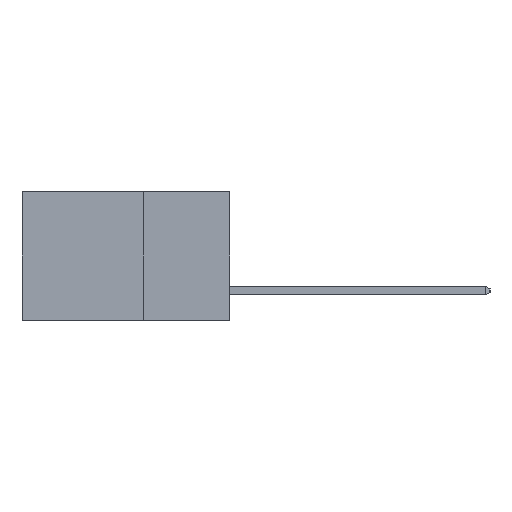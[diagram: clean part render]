
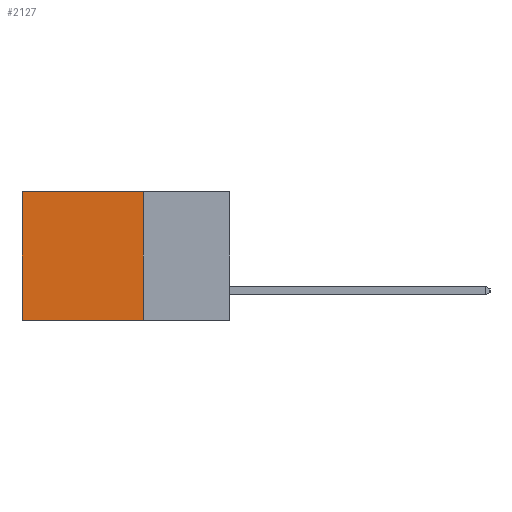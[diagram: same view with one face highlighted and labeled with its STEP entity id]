
A CAD part, left-side view. The second image highlights one B-rep face of the part: STEP entity #2127.
In plain terms, the highlighted planar face has unit normal (-1, 0, 0).
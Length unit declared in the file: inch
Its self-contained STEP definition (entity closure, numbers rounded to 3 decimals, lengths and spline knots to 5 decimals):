
#1116 = EDGE_LOOP ( 'NONE', ( #4929, #5191, #3551, #4195 ) ) ;
#1677 = VERTEX_POINT ( 'NONE', #11367 ) ;
#1803 = EDGE_CURVE ( 'NONE', #4378, #4482, #6108, .T. ) ;
#2127 = ADVANCED_FACE ( 'NONE', ( #8118 ), #7229, .F. ) ;
#2311 = VERTEX_POINT ( 'NONE', #13158 ) ;
#2641 = CARTESIAN_POINT ( 'NONE',  ( 0.298, 0.25, 0. ) ) ;
#3096 = VECTOR ( 'NONE', #8813, 39.37008 ) ;
#3551 = ORIENTED_EDGE ( 'NONE', *, *, #7066, .F. ) ;
#4195 = ORIENTED_EDGE ( 'NONE', *, *, #6946, .T. ) ;
#4280 = DIRECTION ( 'NONE',  ( 0., 1., 0. ) ) ;
#4378 = VERTEX_POINT ( 'NONE', #7848 ) ;
#4402 = CARTESIAN_POINT ( 'NONE',  ( 0.298, 0.6, 0. ) ) ;
#4482 = VERTEX_POINT ( 'NONE', #6864 ) ;
#4929 = ORIENTED_EDGE ( 'NONE', *, *, #8257, .T. ) ;
#5148 = AXIS2_PLACEMENT_3D ( 'NONE', #2641, #12692, #11734 ) ;
#5191 = ORIENTED_EDGE ( 'NONE', *, *, #1803, .F. ) ;
#5741 = VECTOR ( 'NONE', #7874, 39.37008 ) ;
#6108 = LINE ( 'NONE', #10968, #3096 ) ;
#6550 = CARTESIAN_POINT ( 'NONE',  ( 0.298, 0.25, 0. ) ) ;
#6800 = CARTESIAN_POINT ( 'NONE',  ( 0.298, 0.25, 0. ) ) ;
#6864 = CARTESIAN_POINT ( 'NONE',  ( 0.298, 0.6, -0.37 ) ) ;
#6946 = EDGE_CURVE ( 'NONE', #1677, #2311, #8117, .T. ) ;
#7066 = EDGE_CURVE ( 'NONE', #1677, #4378, #8583, .T. ) ;
#7229 = PLANE ( 'NONE',  #5148 ) ;
#7848 = CARTESIAN_POINT ( 'NONE',  ( 0.298, 0.25, -0.37 ) ) ;
#7874 = DIRECTION ( 'NONE',  ( 0., 0., -1. ) ) ;
#8117 = LINE ( 'NONE', #6550, #13006 ) ;
#8118 = FACE_OUTER_BOUND ( 'NONE', #1116, .T. ) ;
#8257 = EDGE_CURVE ( 'NONE', #2311, #4482, #12005, .T. ) ;
#8583 = LINE ( 'NONE', #6800, #5741 ) ;
#8813 = DIRECTION ( 'NONE',  ( 0., 1., 0. ) ) ;
#9194 = VECTOR ( 'NONE', #12941, 39.37008 ) ;
#10968 = CARTESIAN_POINT ( 'NONE',  ( 0.298, 0.25, -0.37 ) ) ;
#11367 = CARTESIAN_POINT ( 'NONE',  ( 0.298, 0.25, 0. ) ) ;
#11734 = DIRECTION ( 'NONE',  ( 0., 0., -1. ) ) ;
#12005 = LINE ( 'NONE', #4402, #9194 ) ;
#12692 = DIRECTION ( 'NONE',  ( 1., 0., 0. ) ) ;
#12941 = DIRECTION ( 'NONE',  ( 0., 0., -1. ) ) ;
#13006 = VECTOR ( 'NONE', #4280, 39.37008 ) ;
#13158 = CARTESIAN_POINT ( 'NONE',  ( 0.298, 0.6, 0. ) ) ;
